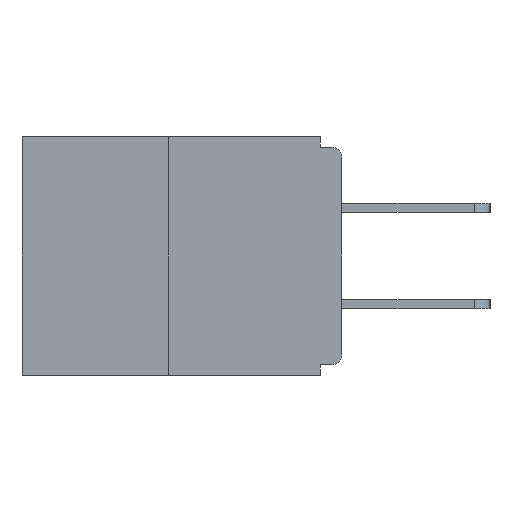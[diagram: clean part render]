
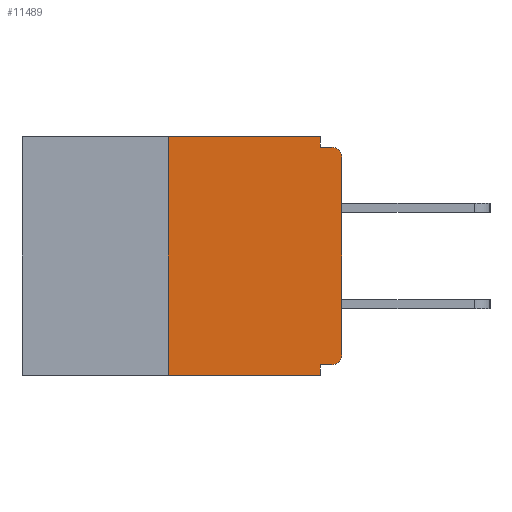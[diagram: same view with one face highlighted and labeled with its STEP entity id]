
A CAD part, left-side view. The second image highlights one B-rep face of the part: STEP entity #11489.
In plain terms, the highlighted planar face has unit normal (-1, 0, 0).
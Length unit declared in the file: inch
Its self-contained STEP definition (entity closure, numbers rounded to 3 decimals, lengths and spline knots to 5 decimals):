
#312 = DIRECTION ( 'NONE',  ( 0., -1., 0. ) ) ;
#610 = DIRECTION ( 'NONE',  ( 0., -1., 0. ) ) ;
#1070 = EDGE_CURVE ( 'NONE', #2963, #5096, #3198, .T. ) ;
#1175 = VECTOR ( 'NONE', #7175, 39.37008 ) ;
#1189 = ORIENTED_EDGE ( 'NONE', *, *, #4924, .T. ) ;
#1269 = CARTESIAN_POINT ( 'NONE',  ( 0., 0.031, -0.343 ) ) ;
#1271 = DIRECTION ( 'NONE',  ( -1., 0., 0. ) ) ;
#1360 = VECTOR ( 'NONE', #3079, 39.37008 ) ;
#1456 = DIRECTION ( 'NONE',  ( 0., -1., 0. ) ) ;
#1483 = DIRECTION ( 'NONE',  ( 0., 0., -1. ) ) ;
#1570 = EDGE_CURVE ( 'NONE', #12112, #4642, #3349, .T. ) ;
#1680 = VECTOR ( 'NONE', #6846, 39.37008 ) ;
#1688 = ORIENTED_EDGE ( 'NONE', *, *, #9118, .T. ) ;
#1998 = ORIENTED_EDGE ( 'NONE', *, *, #5449, .F. ) ;
#2390 = DIRECTION ( 'NONE',  ( 0., 0., -1. ) ) ;
#2445 = LINE ( 'NONE', #3604, #1175 ) ;
#2634 = ORIENTED_EDGE ( 'NONE', *, *, #3254, .F. ) ;
#2963 = VERTEX_POINT ( 'NONE', #10799 ) ;
#3060 = DIRECTION ( 'NONE',  ( 0., 1., 0. ) ) ;
#3079 = DIRECTION ( 'NONE',  ( 0., 0., 1. ) ) ;
#3109 = CIRCLE ( 'NONE', #11347, 0.015 ) ;
#3198 = LINE ( 'NONE', #7424, #13037 ) ;
#3254 = EDGE_CURVE ( 'NONE', #10224, #12112, #12241, .T. ) ;
#3298 = EDGE_CURVE ( 'NONE', #10445, #4936, #9862, .T. ) ;
#3349 = LINE ( 'NONE', #10812, #12665 ) ;
#3482 = DIRECTION ( 'NONE',  ( 0., 0., -1. ) ) ;
#3604 = CARTESIAN_POINT ( 'NONE',  ( 0., 0.031, 0. ) ) ;
#3649 = CARTESIAN_POINT ( 'NONE',  ( 0., 0.46, -0.343 ) ) ;
#4000 = CIRCLE ( 'NONE', #6703, 0.015 ) ;
#4111 = FACE_OUTER_BOUND ( 'NONE', #9232, .T. ) ;
#4336 = LINE ( 'NONE', #11308, #12177 ) ;
#4605 = ORIENTED_EDGE ( 'NONE', *, *, #3298, .F. ) ;
#4642 = VERTEX_POINT ( 'NONE', #10564 ) ;
#4924 = EDGE_CURVE ( 'NONE', #5047, #5096, #4000, .T. ) ;
#4936 = VERTEX_POINT ( 'NONE', #8363 ) ;
#5047 = VERTEX_POINT ( 'NONE', #14316 ) ;
#5096 = VERTEX_POINT ( 'NONE', #10813 ) ;
#5449 = EDGE_CURVE ( 'NONE', #4642, #2963, #2445, .T. ) ;
#5977 = CARTESIAN_POINT ( 'NONE',  ( 0., 0.46, 0. ) ) ;
#6228 = CARTESIAN_POINT ( 'NONE',  ( 0., 0.015, -0.328 ) ) ;
#6392 = VECTOR ( 'NONE', #312, 39.37008 ) ;
#6462 = EDGE_CURVE ( 'NONE', #11332, #5047, #8465, .T. ) ;
#6703 = AXIS2_PLACEMENT_3D ( 'NONE', #7422, #8383, #1483 ) ;
#6789 = VECTOR ( 'NONE', #3482, 39.37008 ) ;
#6846 = DIRECTION ( 'NONE',  ( 0., 0., 1. ) ) ;
#7175 = DIRECTION ( 'NONE',  ( 0., 0., -1. ) ) ;
#7266 = CARTESIAN_POINT ( 'NONE',  ( 0., 0.031, -0.328 ) ) ;
#7422 = CARTESIAN_POINT ( 'NONE',  ( 0., 0.015, -0.03 ) ) ;
#7424 = CARTESIAN_POINT ( 'NONE',  ( 0., 0., -0.015 ) ) ;
#8363 = CARTESIAN_POINT ( 'NONE',  ( 0., 0.031, -0.343 ) ) ;
#8383 = DIRECTION ( 'NONE',  ( -1., 0., 0. ) ) ;
#8465 = LINE ( 'NONE', #10046, #1360 ) ;
#8515 = EDGE_CURVE ( 'NONE', #13833, #11332, #3109, .T. ) ;
#9118 = EDGE_CURVE ( 'NONE', #10224, #4936, #12915, .T. ) ;
#9232 = EDGE_LOOP ( 'NONE', ( #13202, #2634, #1688, #4605, #13608, #10221, #10459, #1189, #12554, #1998 ) ) ;
#9360 = EDGE_CURVE ( 'NONE', #13833, #10445, #4336, .T. ) ;
#9544 = DIRECTION ( 'NONE',  ( 1., 0., 0. ) ) ;
#9629 = DIRECTION ( 'NONE',  ( 0., 0., -1. ) ) ;
#9809 = AXIS2_PLACEMENT_3D ( 'NONE', #5977, #9544, #9629 ) ;
#9862 = LINE ( 'NONE', #1269, #6789 ) ;
#10046 = CARTESIAN_POINT ( 'NONE',  ( 0., 0., 0. ) ) ;
#10123 = CARTESIAN_POINT ( 'NONE',  ( 0., 0.25, -0.343 ) ) ;
#10221 = ORIENTED_EDGE ( 'NONE', *, *, #8515, .T. ) ;
#10224 = VERTEX_POINT ( 'NONE', #10123 ) ;
#10313 = CARTESIAN_POINT ( 'NONE',  ( 0., 0.25, 0. ) ) ;
#10445 = VERTEX_POINT ( 'NONE', #7266 ) ;
#10459 = ORIENTED_EDGE ( 'NONE', *, *, #6462, .T. ) ;
#10564 = CARTESIAN_POINT ( 'NONE',  ( 0., 0.031, 0. ) ) ;
#10576 = CARTESIAN_POINT ( 'NONE',  ( 0., 0.015, -0.313 ) ) ;
#10799 = CARTESIAN_POINT ( 'NONE',  ( 0., 0.031, -0.015 ) ) ;
#10812 = CARTESIAN_POINT ( 'NONE',  ( 0., 0.46, 0. ) ) ;
#10813 = CARTESIAN_POINT ( 'NONE',  ( 0., 0.015, -0.015 ) ) ;
#11308 = CARTESIAN_POINT ( 'NONE',  ( 0., 0., -0.328 ) ) ;
#11332 = VERTEX_POINT ( 'NONE', #14123 ) ;
#11347 = AXIS2_PLACEMENT_3D ( 'NONE', #10576, #1271, #2390 ) ;
#11489 = ADVANCED_FACE ( 'NONE', ( #4111 ), #14201, .F. ) ;
#12112 = VERTEX_POINT ( 'NONE', #10313 ) ;
#12177 = VECTOR ( 'NONE', #3060, 39.37008 ) ;
#12241 = LINE ( 'NONE', #13788, #1680 ) ;
#12554 = ORIENTED_EDGE ( 'NONE', *, *, #1070, .F. ) ;
#12665 = VECTOR ( 'NONE', #1456, 39.37008 ) ;
#12915 = LINE ( 'NONE', #3649, #6392 ) ;
#13037 = VECTOR ( 'NONE', #610, 39.37008 ) ;
#13202 = ORIENTED_EDGE ( 'NONE', *, *, #1570, .F. ) ;
#13608 = ORIENTED_EDGE ( 'NONE', *, *, #9360, .F. ) ;
#13788 = CARTESIAN_POINT ( 'NONE',  ( 0., 0.25, 0. ) ) ;
#13833 = VERTEX_POINT ( 'NONE', #6228 ) ;
#14123 = CARTESIAN_POINT ( 'NONE',  ( 0., 0., -0.313 ) ) ;
#14201 = PLANE ( 'NONE',  #9809 ) ;
#14316 = CARTESIAN_POINT ( 'NONE',  ( 0., 0., -0.03 ) ) ;
